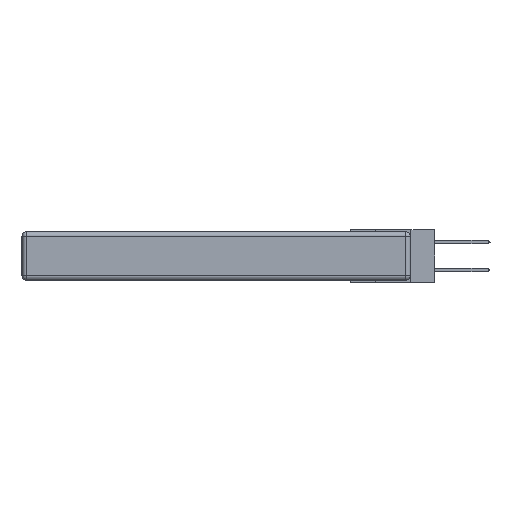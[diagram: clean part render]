
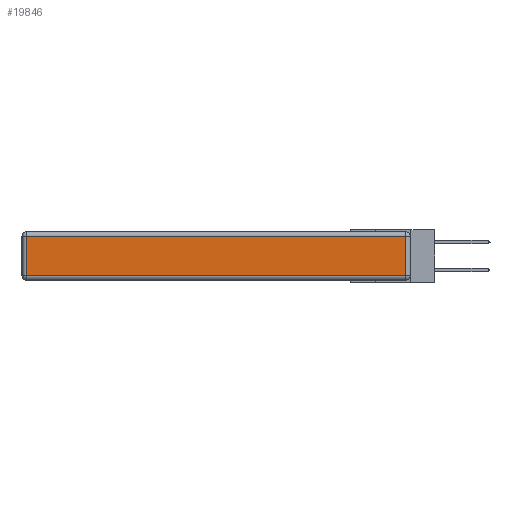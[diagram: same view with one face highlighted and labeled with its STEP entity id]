
A CAD part, left-side view. The second image highlights one B-rep face of the part: STEP entity #19846.
In plain terms, the highlighted planar face has unit normal (-1, 0, 0).
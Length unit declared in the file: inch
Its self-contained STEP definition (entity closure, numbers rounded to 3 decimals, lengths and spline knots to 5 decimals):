
#402 = ORIENTED_EDGE ( 'NONE', *, *, #17907, .T. ) ;
#982 = DIRECTION ( 'NONE',  ( 0., 1., 0. ) ) ;
#1017 = VERTEX_POINT ( 'NONE', #17021 ) ;
#1784 = LINE ( 'NONE', #18166, #6798 ) ;
#2032 = DIRECTION ( 'NONE',  ( 0., 0., 1. ) ) ;
#2100 = VECTOR ( 'NONE', #982, 39.37008 ) ;
#2129 = DIRECTION ( 'NONE',  ( 0., -1., 0. ) ) ;
#4153 = ORIENTED_EDGE ( 'NONE', *, *, #15637, .T. ) ;
#4526 = DIRECTION ( 'NONE',  ( -1., 0., 0. ) ) ;
#5070 = CARTESIAN_POINT ( 'NONE',  ( 0., 0.03, -0.343 ) ) ;
#5117 = ORIENTED_EDGE ( 'NONE', *, *, #10178, .T. ) ;
#5130 = CARTESIAN_POINT ( 'NONE',  ( 0., 2.72, -0.03 ) ) ;
#6150 = DIRECTION ( 'NONE',  ( 0., 0., 1. ) ) ;
#6798 = VECTOR ( 'NONE', #8634, 39.37008 ) ;
#7479 = VECTOR ( 'NONE', #2032, 39.37008 ) ;
#7503 = FACE_OUTER_BOUND ( 'NONE', #18046, .T. ) ;
#8634 = DIRECTION ( 'NONE',  ( 0., 0., -1. ) ) ;
#10178 = EDGE_CURVE ( 'NONE', #19090, #16900, #1784, .T. ) ;
#10337 = LINE ( 'NONE', #16873, #2100 ) ;
#11238 = CARTESIAN_POINT ( 'NONE',  ( 0., 0.03, -0.313 ) ) ;
#13834 = EDGE_CURVE ( 'NONE', #16900, #15271, #19473, .T. ) ;
#14062 = PLANE ( 'NONE',  #14599 ) ;
#14599 = AXIS2_PLACEMENT_3D ( 'NONE', #15641, #4526, #6150 ) ;
#14754 = CARTESIAN_POINT ( 'NONE',  ( 0., 0., -0.313 ) ) ;
#14797 = ORIENTED_EDGE ( 'NONE', *, *, #13834, .T. ) ;
#15049 = CARTESIAN_POINT ( 'NONE',  ( 0., 2.72, -0.313 ) ) ;
#15218 = VECTOR ( 'NONE', #2129, 39.37008 ) ;
#15271 = VERTEX_POINT ( 'NONE', #11238 ) ;
#15637 = EDGE_CURVE ( 'NONE', #15271, #1017, #15911, .T. ) ;
#15641 = CARTESIAN_POINT ( 'NONE',  ( 0., 0., -0.343 ) ) ;
#15911 = LINE ( 'NONE', #5070, #7479 ) ;
#16873 = CARTESIAN_POINT ( 'NONE',  ( 0., 2.75, -0.03 ) ) ;
#16900 = VERTEX_POINT ( 'NONE', #15049 ) ;
#17021 = CARTESIAN_POINT ( 'NONE',  ( 0., 0.03, -0.03 ) ) ;
#17907 = EDGE_CURVE ( 'NONE', #1017, #19090, #10337, .T. ) ;
#18046 = EDGE_LOOP ( 'NONE', ( #14797, #4153, #402, #5117 ) ) ;
#18166 = CARTESIAN_POINT ( 'NONE',  ( 0., 2.72, -0.343 ) ) ;
#19090 = VERTEX_POINT ( 'NONE', #5130 ) ;
#19473 = LINE ( 'NONE', #14754, #15218 ) ;
#19846 = ADVANCED_FACE ( 'NONE', ( #7503 ), #14062, .T. ) ;
